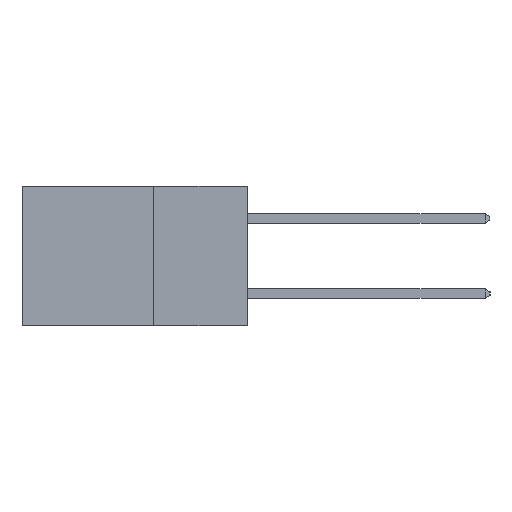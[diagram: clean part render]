
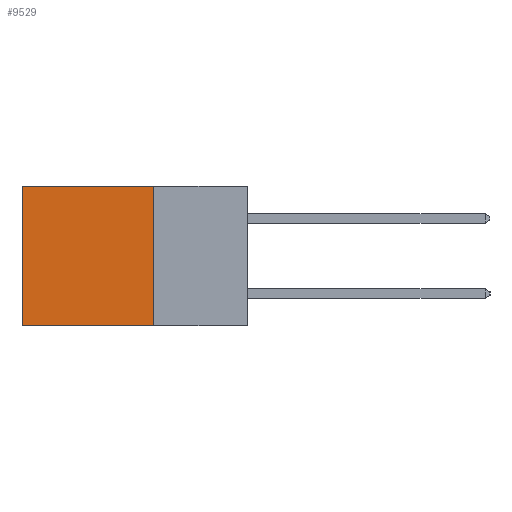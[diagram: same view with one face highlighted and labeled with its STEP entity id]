
A CAD part, left-side view. The second image highlights one B-rep face of the part: STEP entity #9529.
In plain terms, the highlighted planar face has unit normal (-1, 0, 0).
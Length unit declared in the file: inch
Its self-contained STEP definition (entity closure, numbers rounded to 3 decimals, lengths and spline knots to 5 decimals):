
#718 = AXIS2_PLACEMENT_3D ( 'NONE', #2055, #18184, #6180 ) ;
#1554 = CARTESIAN_POINT ( 'NONE',  ( 0.2615, 0.25, -0.37 ) ) ;
#1704 = DIRECTION ( 'NONE',  ( 0., 1., 0. ) ) ;
#2055 = CARTESIAN_POINT ( 'NONE',  ( 0.2615, 0.25, -0.37 ) ) ;
#2582 = VERTEX_POINT ( 'NONE', #8323 ) ;
#2796 = CARTESIAN_POINT ( 'NONE',  ( 0.2615, 0.25, -0.37 ) ) ;
#4283 = VECTOR ( 'NONE', #1704, 39.37008 ) ;
#4419 = VERTEX_POINT ( 'NONE', #22005 ) ;
#4464 = CARTESIAN_POINT ( 'NONE',  ( 0.2615, 0.25, 0. ) ) ;
#4716 = VERTEX_POINT ( 'NONE', #18888 ) ;
#5697 = LINE ( 'NONE', #4464, #21108 ) ;
#5702 = EDGE_LOOP ( 'NONE', ( #6913, #16306, #17155, #22676 ) ) ;
#6180 = DIRECTION ( 'NONE',  ( 0., 0., -1. ) ) ;
#6241 = LINE ( 'NONE', #2796, #16274 ) ;
#6535 = DIRECTION ( 'NONE',  ( 0., 1., 0. ) ) ;
#6913 = ORIENTED_EDGE ( 'NONE', *, *, #23810, .T. ) ;
#7577 = EDGE_CURVE ( 'NONE', #2582, #4419, #20344, .T. ) ;
#7676 = LINE ( 'NONE', #8824, #17680 ) ;
#8067 = FACE_OUTER_BOUND ( 'NONE', #5702, .T. ) ;
#8323 = CARTESIAN_POINT ( 'NONE',  ( 0.2615, 0.25, -0.37 ) ) ;
#8824 = CARTESIAN_POINT ( 'NONE',  ( 0.2615, 0.6, -0.37 ) ) ;
#9529 = ADVANCED_FACE ( 'NONE', ( #8067 ), #24158, .F. ) ;
#10839 = DIRECTION ( 'NONE',  ( 0., 0., -1. ) ) ;
#11606 = EDGE_CURVE ( 'NONE', #13164, #4716, #5697, .T. ) ;
#13164 = VERTEX_POINT ( 'NONE', #23765 ) ;
#16274 = VECTOR ( 'NONE', #18896, 39.37008 ) ;
#16306 = ORIENTED_EDGE ( 'NONE', *, *, #7577, .F. ) ;
#16968 = EDGE_CURVE ( 'NONE', #13164, #2582, #6241, .T. ) ;
#17155 = ORIENTED_EDGE ( 'NONE', *, *, #16968, .F. ) ;
#17680 = VECTOR ( 'NONE', #10839, 39.37008 ) ;
#18184 = DIRECTION ( 'NONE',  ( 1., 0., 0. ) ) ;
#18888 = CARTESIAN_POINT ( 'NONE',  ( 0.2615, 0.6, 0. ) ) ;
#18896 = DIRECTION ( 'NONE',  ( 0., 0., -1. ) ) ;
#20344 = LINE ( 'NONE', #1554, #4283 ) ;
#21108 = VECTOR ( 'NONE', #6535, 39.37008 ) ;
#22005 = CARTESIAN_POINT ( 'NONE',  ( 0.2615, 0.6, -0.37 ) ) ;
#22676 = ORIENTED_EDGE ( 'NONE', *, *, #11606, .T. ) ;
#23765 = CARTESIAN_POINT ( 'NONE',  ( 0.2615, 0.25, 0. ) ) ;
#23810 = EDGE_CURVE ( 'NONE', #4716, #4419, #7676, .T. ) ;
#24158 = PLANE ( 'NONE',  #718 ) ;
